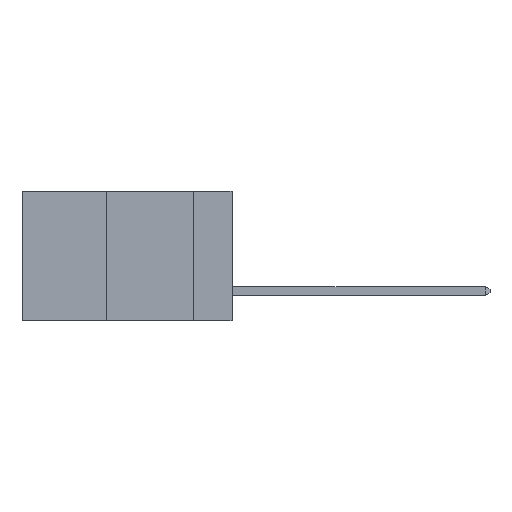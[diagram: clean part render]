
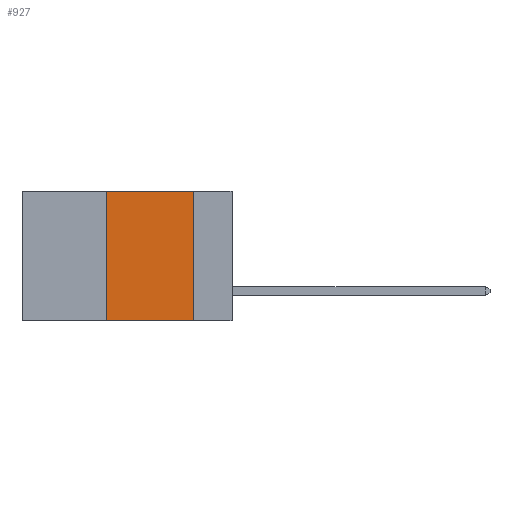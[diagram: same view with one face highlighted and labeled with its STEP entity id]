
A CAD part, left-side view. The second image highlights one B-rep face of the part: STEP entity #927.
In plain terms, the highlighted planar face has unit normal (-1, 0, 0).
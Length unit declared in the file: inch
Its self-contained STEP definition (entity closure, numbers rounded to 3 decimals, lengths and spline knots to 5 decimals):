
#37 = CARTESIAN_POINT ( 'NONE',  ( 0., 0.36, 0. ) ) ;
#800 = ORIENTED_EDGE ( 'NONE', *, *, #1851, .T. ) ;
#927 = ADVANCED_FACE ( 'NONE', ( #22640 ), #1273, .F. ) ;
#1273 = PLANE ( 'NONE',  #15352 ) ;
#1314 = CARTESIAN_POINT ( 'NONE',  ( 0., 0.6, 0. ) ) ;
#1368 = DIRECTION ( 'NONE',  ( 1., 0., 0. ) ) ;
#1424 = DIRECTION ( 'NONE',  ( 0., 0., -1. ) ) ;
#1594 = VECTOR ( 'NONE', #2092, 39.37008 ) ;
#1851 = EDGE_CURVE ( 'NONE', #11804, #22619, #21806, .T. ) ;
#2092 = DIRECTION ( 'NONE',  ( 0., 0., -1. ) ) ;
#2138 = CARTESIAN_POINT ( 'NONE',  ( 0., 0.11, 0. ) ) ;
#2173 = LINE ( 'NONE', #13039, #1594 ) ;
#2284 = LINE ( 'NONE', #9428, #21000 ) ;
#3852 = EDGE_CURVE ( 'NONE', #4565, #22619, #2173, .T. ) ;
#3875 = DIRECTION ( 'NONE',  ( 0., -1., 0. ) ) ;
#4565 = VERTEX_POINT ( 'NONE', #2138 ) ;
#4598 = ORIENTED_EDGE ( 'NONE', *, *, #3852, .F. ) ;
#6502 = EDGE_LOOP ( 'NONE', ( #4598, #14239, #19617, #800 ) ) ;
#7604 = DIRECTION ( 'NONE',  ( 0., -1., 0. ) ) ;
#7828 = EDGE_CURVE ( 'NONE', #11804, #13511, #12972, .T. ) ;
#9428 = CARTESIAN_POINT ( 'NONE',  ( 0., 0.6, 0. ) ) ;
#11034 = CARTESIAN_POINT ( 'NONE',  ( 0., 0.6, -0.37 ) ) ;
#11739 = CARTESIAN_POINT ( 'NONE',  ( 0., 0.11, -0.37 ) ) ;
#11804 = VERTEX_POINT ( 'NONE', #22185 ) ;
#12972 = LINE ( 'NONE', #19782, #21919 ) ;
#13039 = CARTESIAN_POINT ( 'NONE',  ( 0., 0.11, 0. ) ) ;
#13511 = VERTEX_POINT ( 'NONE', #37 ) ;
#14229 = EDGE_CURVE ( 'NONE', #13511, #4565, #2284, .T. ) ;
#14239 = ORIENTED_EDGE ( 'NONE', *, *, #14229, .F. ) ;
#15352 = AXIS2_PLACEMENT_3D ( 'NONE', #1314, #1368, #1424 ) ;
#17066 = VECTOR ( 'NONE', #7604, 39.37008 ) ;
#19617 = ORIENTED_EDGE ( 'NONE', *, *, #7828, .F. ) ;
#19782 = CARTESIAN_POINT ( 'NONE',  ( 0., 0.36, 0. ) ) ;
#21000 = VECTOR ( 'NONE', #3875, 39.37008 ) ;
#21806 = LINE ( 'NONE', #11034, #17066 ) ;
#21919 = VECTOR ( 'NONE', #23295, 39.37008 ) ;
#22185 = CARTESIAN_POINT ( 'NONE',  ( 0., 0.36, -0.37 ) ) ;
#22619 = VERTEX_POINT ( 'NONE', #11739 ) ;
#22640 = FACE_OUTER_BOUND ( 'NONE', #6502, .T. ) ;
#23295 = DIRECTION ( 'NONE',  ( 0., 0., 1. ) ) ;
